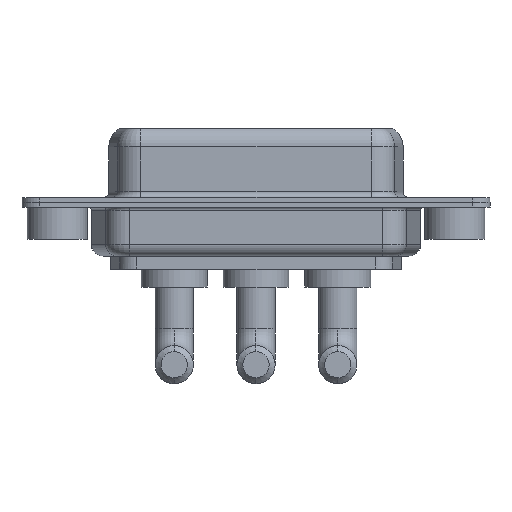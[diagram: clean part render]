
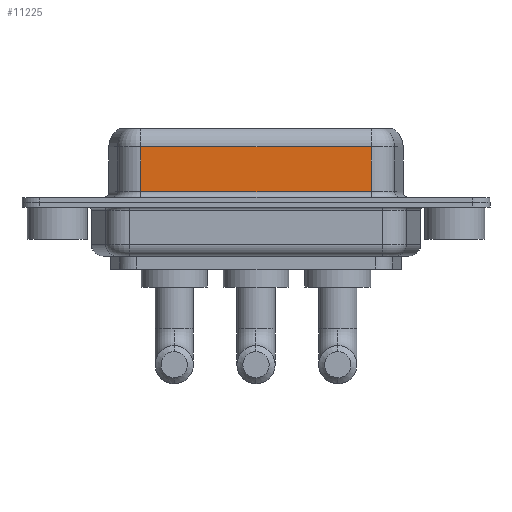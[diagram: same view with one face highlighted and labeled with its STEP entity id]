
A CAD part, front view. The second image highlights one B-rep face of the part: STEP entity #11225.
In plain terms, the highlighted planar face has unit normal (0, -1, 0).
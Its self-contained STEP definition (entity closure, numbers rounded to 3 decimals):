
#173 = ORIENTED_EDGE ( 'NONE', *, *, #6810, .T. ) ;
#330 = LINE ( 'NONE', #4947, #10666 ) ;
#713 = EDGE_CURVE ( 'NONE', #10211, #1427, #1283, .T. ) ;
#830 = CARTESIAN_POINT ( 'NONE',  ( 26.287, -3.95, 0.9 ) ) ;
#1037 = DIRECTION ( 'NONE',  ( 0., 1., 0. ) ) ;
#1232 = VECTOR ( 'NONE', #1572, 1000. ) ;
#1283 = LINE ( 'NONE', #10743, #4739 ) ;
#1427 = VERTEX_POINT ( 'NONE', #830 ) ;
#1572 = DIRECTION ( 'NONE',  ( 0., 0., -1. ) ) ;
#1586 = EDGE_LOOP ( 'NONE', ( #10586, #2328, #173, #5828 ) ) ;
#2328 = ORIENTED_EDGE ( 'NONE', *, *, #6523, .T. ) ;
#2531 = LINE ( 'NONE', #6303, #1232 ) ;
#3023 = VECTOR ( 'NONE', #8640, 1000. ) ;
#3905 = DIRECTION ( 'NONE',  ( 0., 0., 1. ) ) ;
#4739 = VECTOR ( 'NONE', #8137, 1000. ) ;
#4834 = LINE ( 'NONE', #12302, #3023 ) ;
#4947 = CARTESIAN_POINT ( 'NONE',  ( 26.287, -3.95, 0.9 ) ) ;
#5148 = CARTESIAN_POINT ( 'NONE',  ( 7.013, -3.95, 4.65 ) ) ;
#5828 = ORIENTED_EDGE ( 'NONE', *, *, #10044, .T. ) ;
#6303 = CARTESIAN_POINT ( 'NONE',  ( 7.013, -3.95, 6.4 ) ) ;
#6461 = FACE_OUTER_BOUND ( 'NONE', #1586, .T. ) ;
#6523 = EDGE_CURVE ( 'NONE', #10211, #10816, #4834, .T. ) ;
#6810 = EDGE_CURVE ( 'NONE', #10816, #10542, #2531, .T. ) ;
#7641 = AXIS2_PLACEMENT_3D ( 'NONE', #7647, #1037, #3905 ) ;
#7647 = CARTESIAN_POINT ( 'NONE',  ( 26.287, -3.95, 6.4 ) ) ;
#8137 = DIRECTION ( 'NONE',  ( 0., 0., -1. ) ) ;
#8357 = CARTESIAN_POINT ( 'NONE',  ( 7.013, -3.95, 0.9 ) ) ;
#8640 = DIRECTION ( 'NONE',  ( -1., 0., 0. ) ) ;
#8821 = DIRECTION ( 'NONE',  ( 1., 0., 0. ) ) ;
#9185 = CARTESIAN_POINT ( 'NONE',  ( 26.287, -3.95, 4.65 ) ) ;
#10044 = EDGE_CURVE ( 'NONE', #10542, #1427, #330, .T. ) ;
#10211 = VERTEX_POINT ( 'NONE', #9185 ) ;
#10542 = VERTEX_POINT ( 'NONE', #8357 ) ;
#10586 = ORIENTED_EDGE ( 'NONE', *, *, #713, .F. ) ;
#10666 = VECTOR ( 'NONE', #8821, 1000. ) ;
#10743 = CARTESIAN_POINT ( 'NONE',  ( 26.287, -3.95, 6.4 ) ) ;
#10816 = VERTEX_POINT ( 'NONE', #5148 ) ;
#11225 = ADVANCED_FACE ( 'NONE', ( #6461 ), #12248, .F. ) ;
#12248 = PLANE ( 'NONE',  #7641 ) ;
#12302 = CARTESIAN_POINT ( 'NONE',  ( 26.287, -3.95, 4.65 ) ) ;
